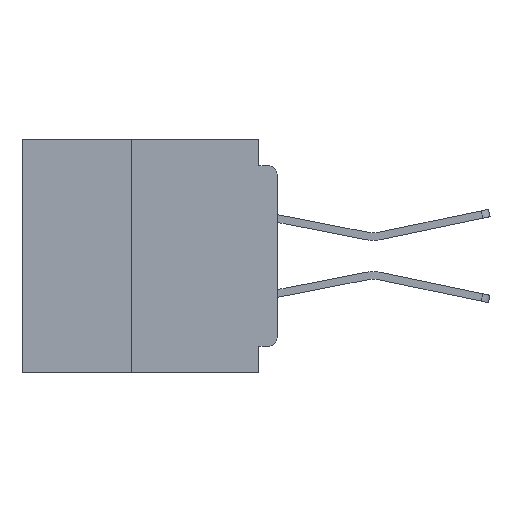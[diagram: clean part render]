
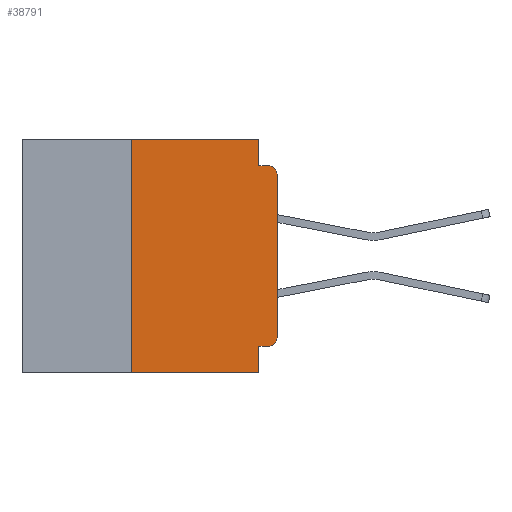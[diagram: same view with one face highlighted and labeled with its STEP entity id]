
A CAD part, left-side view. The second image highlights one B-rep face of the part: STEP entity #38791.
In plain terms, the highlighted planar face has unit normal (-1, 0, 0).
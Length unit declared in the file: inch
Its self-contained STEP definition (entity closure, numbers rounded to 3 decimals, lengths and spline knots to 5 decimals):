
#58 = ORIENTED_EDGE ( 'NONE', *, *, #39548, .T. ) ;
#1090 = ORIENTED_EDGE ( 'NONE', *, *, #33873, .T. ) ;
#1603 = CARTESIAN_POINT ( 'NONE',  ( 0., 0.015, -0.355 ) ) ;
#1832 = DIRECTION ( 'NONE',  ( 0., 0., 1. ) ) ;
#3207 = DIRECTION ( 'NONE',  ( -1., 0., 0. ) ) ;
#3540 = ORIENTED_EDGE ( 'NONE', *, *, #25859, .F. ) ;
#4275 = LINE ( 'NONE', #18652, #15781 ) ;
#4654 = CARTESIAN_POINT ( 'NONE',  ( 0., 0., -0.355 ) ) ;
#6815 = EDGE_CURVE ( 'NONE', #50002, #30072, #18691, .T. ) ;
#8503 = EDGE_CURVE ( 'NONE', #30072, #14499, #37619, .T. ) ;
#8838 = DIRECTION ( 'NONE',  ( 0., -1., 0. ) ) ;
#9835 = CARTESIAN_POINT ( 'NONE',  ( 0., 0.031, -0.355 ) ) ;
#10877 = AXIS2_PLACEMENT_3D ( 'NONE', #29062, #3207, #33331 ) ;
#11213 = EDGE_LOOP ( 'NONE', ( #13049, #1090, #42228, #3540, #15794, #49870, #21067, #42474, #35662, #58 ) ) ;
#12855 = AXIS2_PLACEMENT_3D ( 'NONE', #43133, #55293, #30090 ) ;
#13049 = ORIENTED_EDGE ( 'NONE', *, *, #45911, .T. ) ;
#13466 = VECTOR ( 'NONE', #54431, 39.37008 ) ;
#13795 = VECTOR ( 'NONE', #24806, 39.37008 ) ;
#14499 = VERTEX_POINT ( 'NONE', #25535 ) ;
#15781 = VECTOR ( 'NONE', #52566, 39.37008 ) ;
#15794 = ORIENTED_EDGE ( 'NONE', *, *, #45652, .F. ) ;
#16278 = VERTEX_POINT ( 'NONE', #39930 ) ;
#16968 = CARTESIAN_POINT ( 'NONE',  ( 0., 0.437, 0. ) ) ;
#18652 = CARTESIAN_POINT ( 'NONE',  ( 0., 0.031, 0. ) ) ;
#18678 = LINE ( 'NONE', #51216, #51226 ) ;
#18691 = LINE ( 'NONE', #4654, #40073 ) ;
#18974 = DIRECTION ( 'NONE',  ( 0., -1., 0. ) ) ;
#20080 = EDGE_CURVE ( 'NONE', #39256, #14499, #42435, .T. ) ;
#21067 = ORIENTED_EDGE ( 'NONE', *, *, #20080, .T. ) ;
#21073 = CARTESIAN_POINT ( 'NONE',  ( 0., 0.031, 0. ) ) ;
#21405 = CARTESIAN_POINT ( 'NONE',  ( 0., 0.031, -0.045 ) ) ;
#21927 = CARTESIAN_POINT ( 'NONE',  ( 0., 0.015, -0.34 ) ) ;
#24408 = VERTEX_POINT ( 'NONE', #21073 ) ;
#24630 = CARTESIAN_POINT ( 'NONE',  ( 0., 0.25, 0. ) ) ;
#24806 = DIRECTION ( 'NONE',  ( 0., -1., 0. ) ) ;
#25535 = CARTESIAN_POINT ( 'NONE',  ( 0., 0.031, -0.4 ) ) ;
#25859 = EDGE_CURVE ( 'NONE', #24408, #33367, #4275, .T. ) ;
#26231 = DIRECTION ( 'NONE',  ( 0., 0., -1. ) ) ;
#27673 = CARTESIAN_POINT ( 'NONE',  ( 0., 0., 0. ) ) ;
#28056 = AXIS2_PLACEMENT_3D ( 'NONE', #21927, #51557, #26231 ) ;
#29062 = CARTESIAN_POINT ( 'NONE',  ( 0., 0.015, -0.06 ) ) ;
#29338 = CARTESIAN_POINT ( 'NONE',  ( 0., 0., -0.045 ) ) ;
#30072 = VERTEX_POINT ( 'NONE', #9835 ) ;
#30090 = DIRECTION ( 'NONE',  ( 0., 0., -1. ) ) ;
#31190 = VECTOR ( 'NONE', #18974, 39.37008 ) ;
#32003 = VERTEX_POINT ( 'NONE', #24630 ) ;
#32748 = VERTEX_POINT ( 'NONE', #54875 ) ;
#33331 = DIRECTION ( 'NONE',  ( 0., 0., -1. ) ) ;
#33367 = VERTEX_POINT ( 'NONE', #21405 ) ;
#33469 = CARTESIAN_POINT ( 'NONE',  ( 0., 0.031, -0.4 ) ) ;
#33854 = FACE_OUTER_BOUND ( 'NONE', #11213, .T. ) ;
#33873 = EDGE_CURVE ( 'NONE', #16278, #43397, #52748, .T. ) ;
#34371 = VECTOR ( 'NONE', #8838, 39.37008 ) ;
#34761 = DIRECTION ( 'NONE',  ( 0., 1., 0. ) ) ;
#35013 = VECTOR ( 'NONE', #1832, 39.37008 ) ;
#35662 = ORIENTED_EDGE ( 'NONE', *, *, #6815, .F. ) ;
#35692 = LINE ( 'NONE', #16968, #34371 ) ;
#37078 = CARTESIAN_POINT ( 'NONE',  ( 0., 0.25, -0.4 ) ) ;
#37619 = LINE ( 'NONE', #33469, #13466 ) ;
#38570 = DIRECTION ( 'NONE',  ( 0., 0., 1. ) ) ;
#38791 = ADVANCED_FACE ( 'NONE', ( #33854 ), #51814, .F. ) ;
#39256 = VERTEX_POINT ( 'NONE', #37078 ) ;
#39548 = EDGE_CURVE ( 'NONE', #50002, #32748, #51524, .T. ) ;
#39930 = CARTESIAN_POINT ( 'NONE',  ( 0., 0., -0.06 ) ) ;
#40073 = VECTOR ( 'NONE', #34761, 39.37008 ) ;
#40277 = CARTESIAN_POINT ( 'NONE',  ( 0., 0.437, -0.4 ) ) ;
#42228 = ORIENTED_EDGE ( 'NONE', *, *, #49739, .F. ) ;
#42435 = LINE ( 'NONE', #40277, #31190 ) ;
#42474 = ORIENTED_EDGE ( 'NONE', *, *, #8503, .F. ) ;
#43133 = CARTESIAN_POINT ( 'NONE',  ( 0., 0.437, 0. ) ) ;
#43397 = VERTEX_POINT ( 'NONE', #45120 ) ;
#44348 = LINE ( 'NONE', #27673, #35013 ) ;
#45120 = CARTESIAN_POINT ( 'NONE',  ( 0., 0.015, -0.045 ) ) ;
#45652 = EDGE_CURVE ( 'NONE', #32003, #24408, #35692, .T. ) ;
#45911 = EDGE_CURVE ( 'NONE', #32748, #16278, #44348, .T. ) ;
#47821 = LINE ( 'NONE', #29338, #13795 ) ;
#48574 = EDGE_CURVE ( 'NONE', #39256, #32003, #18678, .T. ) ;
#49739 = EDGE_CURVE ( 'NONE', #33367, #43397, #47821, .T. ) ;
#49870 = ORIENTED_EDGE ( 'NONE', *, *, #48574, .F. ) ;
#50002 = VERTEX_POINT ( 'NONE', #1603 ) ;
#51216 = CARTESIAN_POINT ( 'NONE',  ( 0., 0.25, -0.4 ) ) ;
#51226 = VECTOR ( 'NONE', #38570, 39.37008 ) ;
#51524 = CIRCLE ( 'NONE', #28056, 0.015 ) ;
#51557 = DIRECTION ( 'NONE',  ( -1., 0., 0. ) ) ;
#51814 = PLANE ( 'NONE',  #12855 ) ;
#52566 = DIRECTION ( 'NONE',  ( 0., 0., -1. ) ) ;
#52748 = CIRCLE ( 'NONE', #10877, 0.015 ) ;
#54431 = DIRECTION ( 'NONE',  ( 0., 0., -1. ) ) ;
#54875 = CARTESIAN_POINT ( 'NONE',  ( 0., 0., -0.34 ) ) ;
#55293 = DIRECTION ( 'NONE',  ( 1., 0., 0. ) ) ;
